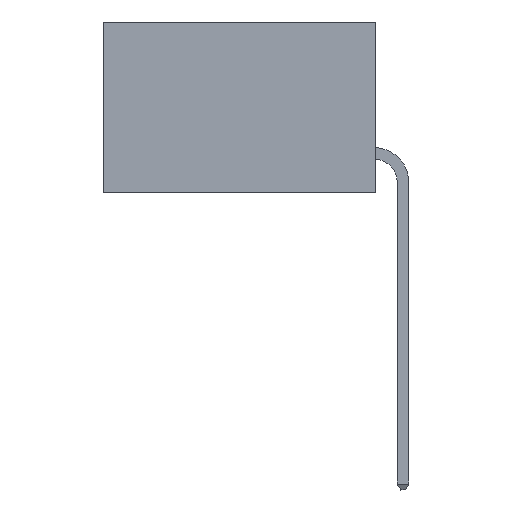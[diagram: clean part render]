
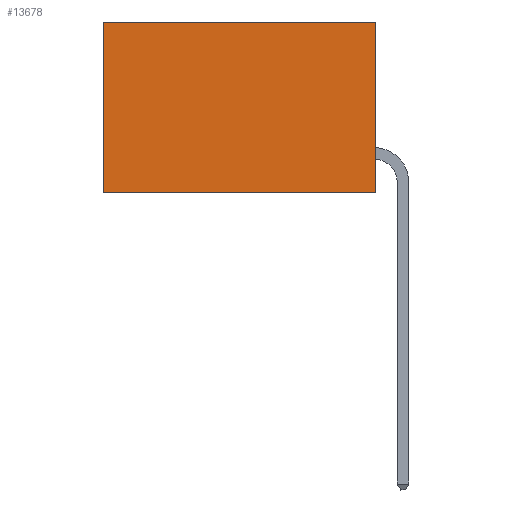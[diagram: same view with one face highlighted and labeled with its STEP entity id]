
A CAD part, left-side view. The second image highlights one B-rep face of the part: STEP entity #13678.
In plain terms, the highlighted planar face has unit normal (-1, 0, 0).
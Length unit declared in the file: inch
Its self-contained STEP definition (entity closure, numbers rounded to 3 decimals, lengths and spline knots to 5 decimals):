
#648 = VECTOR ( 'NONE', #14178, 39.37008 ) ;
#1212 = ORIENTED_EDGE ( 'NONE', *, *, #14660, .T. ) ;
#2767 = LINE ( 'NONE', #23337, #22135 ) ;
#3109 = VERTEX_POINT ( 'NONE', #13711 ) ;
#3126 = DIRECTION ( 'NONE',  ( 0., 1., 0. ) ) ;
#3343 = FACE_OUTER_BOUND ( 'NONE', #5166, .T. ) ;
#3553 = ORIENTED_EDGE ( 'NONE', *, *, #12385, .T. ) ;
#3685 = PLANE ( 'NONE',  #30572 ) ;
#5166 = EDGE_LOOP ( 'NONE', ( #3553, #27207, #31054, #1212 ) ) ;
#5560 = DIRECTION ( 'NONE',  ( 0., 1., 0. ) ) ;
#6241 = DIRECTION ( 'NONE',  ( 0., 0., -1. ) ) ;
#7274 = EDGE_CURVE ( 'NONE', #18264, #19767, #30471, .T. ) ;
#8302 = VERTEX_POINT ( 'NONE', #30386 ) ;
#11746 = VECTOR ( 'NONE', #5560, 39.37008 ) ;
#12385 = EDGE_CURVE ( 'NONE', #3109, #8302, #15681, .T. ) ;
#13678 = ADVANCED_FACE ( 'NONE', ( #3343 ), #3685, .F. ) ;
#13711 = CARTESIAN_POINT ( 'NONE',  ( 0.277, 0.59, 0. ) ) ;
#14178 = DIRECTION ( 'NONE',  ( 0., 0., -1. ) ) ;
#14660 = EDGE_CURVE ( 'NONE', #18264, #3109, #18458, .T. ) ;
#15681 = LINE ( 'NONE', #24192, #648 ) ;
#18264 = VERTEX_POINT ( 'NONE', #27242 ) ;
#18431 = DIRECTION ( 'NONE',  ( 0., 0., -1. ) ) ;
#18458 = LINE ( 'NONE', #28134, #11746 ) ;
#19767 = VERTEX_POINT ( 'NONE', #25529 ) ;
#20485 = EDGE_CURVE ( 'NONE', #19767, #8302, #2767, .T. ) ;
#21373 = DIRECTION ( 'NONE',  ( 1., 0., 0. ) ) ;
#22135 = VECTOR ( 'NONE', #3126, 39.37008 ) ;
#23337 = CARTESIAN_POINT ( 'NONE',  ( 0.277, 0., -0.37 ) ) ;
#23857 = VECTOR ( 'NONE', #18431, 39.37008 ) ;
#24192 = CARTESIAN_POINT ( 'NONE',  ( 0.277, 0.59, -0.37 ) ) ;
#25529 = CARTESIAN_POINT ( 'NONE',  ( 0.277, 0., -0.37 ) ) ;
#26315 = CARTESIAN_POINT ( 'NONE',  ( 0.277, 0., -0.37 ) ) ;
#27207 = ORIENTED_EDGE ( 'NONE', *, *, #20485, .F. ) ;
#27242 = CARTESIAN_POINT ( 'NONE',  ( 0.277, 0., 0. ) ) ;
#28134 = CARTESIAN_POINT ( 'NONE',  ( 0.277, 0., 0. ) ) ;
#28396 = CARTESIAN_POINT ( 'NONE',  ( 0.277, 0., -0.37 ) ) ;
#30386 = CARTESIAN_POINT ( 'NONE',  ( 0.277, 0.59, -0.37 ) ) ;
#30471 = LINE ( 'NONE', #28396, #23857 ) ;
#30572 = AXIS2_PLACEMENT_3D ( 'NONE', #26315, #21373, #6241 ) ;
#31054 = ORIENTED_EDGE ( 'NONE', *, *, #7274, .F. ) ;
